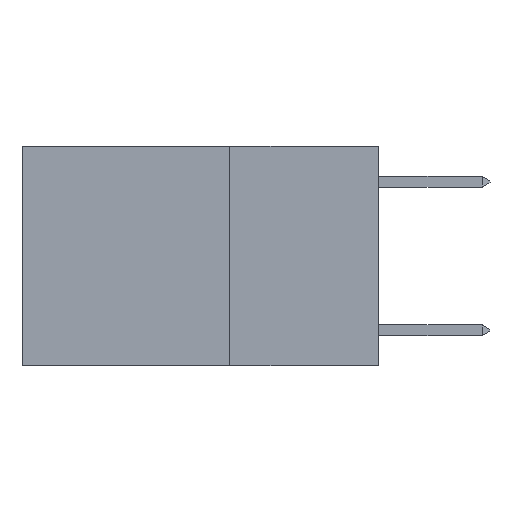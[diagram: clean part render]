
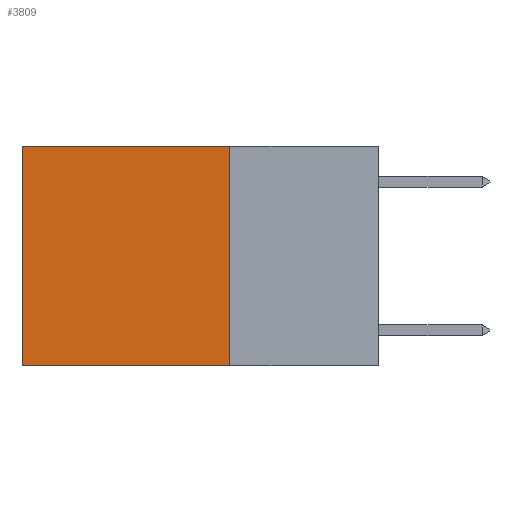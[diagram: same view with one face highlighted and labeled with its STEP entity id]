
A CAD part, left-side view. The second image highlights one B-rep face of the part: STEP entity #3809.
In plain terms, the highlighted planar face has unit normal (-1, 0, 0).
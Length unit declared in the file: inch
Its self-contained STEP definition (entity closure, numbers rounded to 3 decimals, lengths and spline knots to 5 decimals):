
#803 = DIRECTION ( 'NONE',  ( 0., 1., 0. ) ) ;
#855 = CARTESIAN_POINT ( 'NONE',  ( 0.2625, 0.25, 0. ) ) ;
#1138 = ORIENTED_EDGE ( 'NONE', *, *, #7901, .F. ) ;
#1344 = DIRECTION ( 'NONE',  ( 0., 0., -1. ) ) ;
#1437 = EDGE_CURVE ( 'NONE', #1564, #7507, #5509, .T. ) ;
#1564 = VERTEX_POINT ( 'NONE', #2090 ) ;
#2023 = VERTEX_POINT ( 'NONE', #3503 ) ;
#2044 = DIRECTION ( 'NONE',  ( 0., 0., -1. ) ) ;
#2090 = CARTESIAN_POINT ( 'NONE',  ( 0.2625, 0.25, 0. ) ) ;
#2136 = LINE ( 'NONE', #5322, #4082 ) ;
#2748 = AXIS2_PLACEMENT_3D ( 'NONE', #3677, #6191, #7613 ) ;
#2868 = LINE ( 'NONE', #855, #5958 ) ;
#2915 = EDGE_LOOP ( 'NONE', ( #6566, #1138, #7940, #4474 ) ) ;
#2922 = FACE_OUTER_BOUND ( 'NONE', #2915, .T. ) ;
#3503 = CARTESIAN_POINT ( 'NONE',  ( 0.2625, 0.25, -0.37 ) ) ;
#3677 = CARTESIAN_POINT ( 'NONE',  ( 0.2625, 0.25, 0. ) ) ;
#3809 = ADVANCED_FACE ( 'NONE', ( #2922 ), #4967, .F. ) ;
#3951 = VECTOR ( 'NONE', #803, 39.37008 ) ;
#4020 = DIRECTION ( 'NONE',  ( 0., 1., 0. ) ) ;
#4081 = CARTESIAN_POINT ( 'NONE',  ( 0.2625, 0.6, 0. ) ) ;
#4082 = VECTOR ( 'NONE', #2044, 39.37008 ) ;
#4105 = VECTOR ( 'NONE', #4020, 39.37008 ) ;
#4474 = ORIENTED_EDGE ( 'NONE', *, *, #1437, .T. ) ;
#4776 = VERTEX_POINT ( 'NONE', #5224 ) ;
#4967 = PLANE ( 'NONE',  #2748 ) ;
#5224 = CARTESIAN_POINT ( 'NONE',  ( 0.2625, 0.6, -0.37 ) ) ;
#5322 = CARTESIAN_POINT ( 'NONE',  ( 0.2625, 0.6, 0. ) ) ;
#5323 = CARTESIAN_POINT ( 'NONE',  ( 0.2625, 0.25, 0. ) ) ;
#5509 = LINE ( 'NONE', #5323, #3951 ) ;
#5660 = EDGE_CURVE ( 'NONE', #7507, #4776, #2136, .T. ) ;
#5958 = VECTOR ( 'NONE', #1344, 39.37008 ) ;
#6060 = LINE ( 'NONE', #8162, #4105 ) ;
#6191 = DIRECTION ( 'NONE',  ( 1., 0., 0. ) ) ;
#6566 = ORIENTED_EDGE ( 'NONE', *, *, #5660, .T. ) ;
#6601 = EDGE_CURVE ( 'NONE', #1564, #2023, #2868, .T. ) ;
#7507 = VERTEX_POINT ( 'NONE', #4081 ) ;
#7613 = DIRECTION ( 'NONE',  ( 0., 0., -1. ) ) ;
#7901 = EDGE_CURVE ( 'NONE', #2023, #4776, #6060, .T. ) ;
#7940 = ORIENTED_EDGE ( 'NONE', *, *, #6601, .F. ) ;
#8162 = CARTESIAN_POINT ( 'NONE',  ( 0.2625, 0.25, -0.37 ) ) ;
